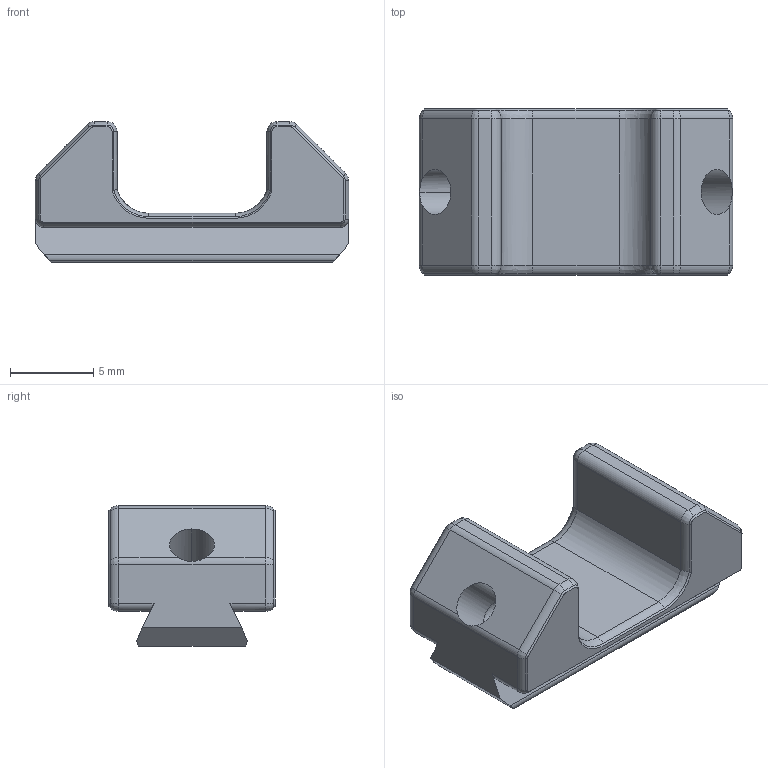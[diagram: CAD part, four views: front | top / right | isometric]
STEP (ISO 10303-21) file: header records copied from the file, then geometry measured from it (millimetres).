
FILE_DESCRIPTION(/* description */ (''),/* implementation_level */ '2;1');
FILE_NAME(/* name */ 'Mount-Locking Block.step',/* time_stamp */ '2021-06-23T22:22:48-04:00',/* author */ (''),/* organization */ (''),/* preprocessor_version */ 'ST-DEVELOPER v18.1',/* originating_system */ 'Autodesk Translation Framework v10.9.0.1377',/* authorisation */ '');
FILE_SCHEMA (('AUTOMOTIVE_DESIGN { 1 0 10303 214 3 1 1 }'));
Length unit declared in the file: millimetre
Products named in the file (1): Mount/Locking Block
Bounding box: 18.8 x 9.97 x 8.45 mm (x, y, z)
Volume: 780.3 mm3; surface area: 833.1 mm2
Topology: 1 solids, 1 shells, 121 faces, 276 edges, 157 vertices
Faces by surface type: plane 42, cylinder 37, bspline 20, cone 20, torus 2
Full cylindrical faces by diameter (mm): 2.7 x1
Entity records: 3619 total; most frequent: CARTESIAN_POINT 921, DIRECTION 567, ORIENTED_EDGE 552, EDGE_CURVE 276, AXIS2_PLACEMENT_3D 209, VERTEX_POINT 157, LINE 149, VECTOR 149
